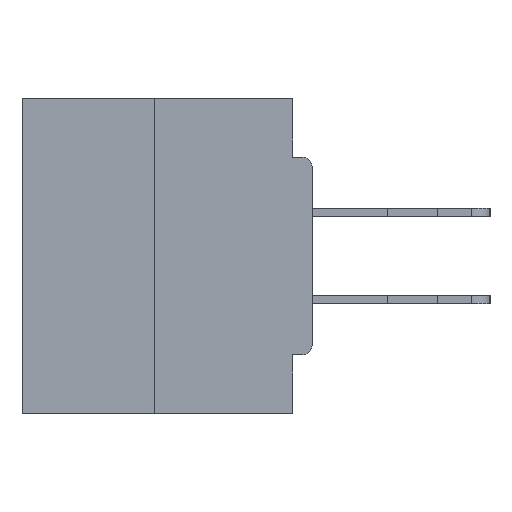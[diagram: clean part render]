
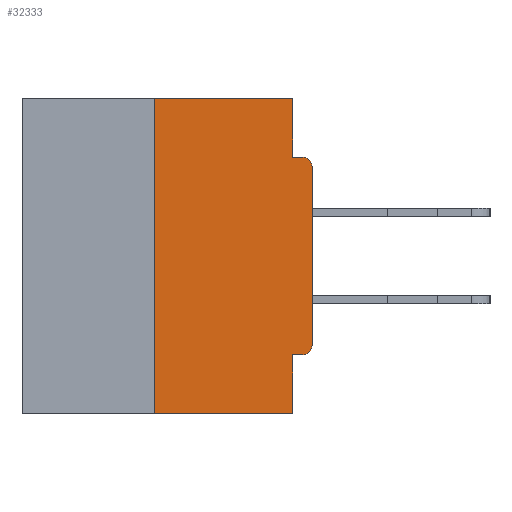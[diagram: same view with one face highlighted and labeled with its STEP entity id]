
A CAD part, left-side view. The second image highlights one B-rep face of the part: STEP entity #32333.
In plain terms, the highlighted planar face has unit normal (-1, 0, 0).
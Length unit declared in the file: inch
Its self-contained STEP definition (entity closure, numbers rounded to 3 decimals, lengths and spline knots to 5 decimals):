
#236 = CARTESIAN_POINT ( 'NONE',  ( 0., 0., -0.3915 ) ) ;
#576 = EDGE_CURVE ( 'NONE', #13654, #20772, #26147, .T. ) ;
#1003 = AXIS2_PLACEMENT_3D ( 'NONE', #36951, #21692, #18489 ) ;
#1049 = DIRECTION ( 'NONE',  ( 0., 0., 1. ) ) ;
#1581 = DIRECTION ( 'NONE',  ( 0., 0., -1. ) ) ;
#1996 = CARTESIAN_POINT ( 'NONE',  ( 0., 0.46, 0. ) ) ;
#2243 = LINE ( 'NONE', #33678, #24818 ) ;
#2298 = CARTESIAN_POINT ( 'NONE',  ( 0., 0.25, -0.5 ) ) ;
#2700 = FACE_OUTER_BOUND ( 'NONE', #12124, .T. ) ;
#2946 = VECTOR ( 'NONE', #6244, 39.37008 ) ;
#3022 = CARTESIAN_POINT ( 'NONE',  ( 0., 0.46, -0.5 ) ) ;
#3078 = LINE ( 'NONE', #3022, #37102 ) ;
#6244 = DIRECTION ( 'NONE',  ( 0., 1., 0. ) ) ;
#6319 = CARTESIAN_POINT ( 'NONE',  ( 0., 0.031, 0. ) ) ;
#6423 = DIRECTION ( 'NONE',  ( 0., 0., -1. ) ) ;
#7347 = CARTESIAN_POINT ( 'NONE',  ( 0., 0.46, 0. ) ) ;
#7908 = ORIENTED_EDGE ( 'NONE', *, *, #17415, .F. ) ;
#8770 = VERTEX_POINT ( 'NONE', #2298 ) ;
#9186 = DIRECTION ( 'NONE',  ( 0., 0., 1. ) ) ;
#9781 = CARTESIAN_POINT ( 'NONE',  ( 0., 0.031, -0.4065 ) ) ;
#10507 = VECTOR ( 'NONE', #1049, 39.37008 ) ;
#10879 = CARTESIAN_POINT ( 'NONE',  ( 0., 0., -0.1085 ) ) ;
#11119 = VECTOR ( 'NONE', #9186, 39.37008 ) ;
#11403 = ORIENTED_EDGE ( 'NONE', *, *, #34003, .F. ) ;
#11912 = CARTESIAN_POINT ( 'NONE',  ( 0., 0., 0. ) ) ;
#12124 = EDGE_LOOP ( 'NONE', ( #12538, #17332, #17091, #23481, #7908, #25326, #17087, #36339, #18971, #11403 ) ) ;
#12354 = CARTESIAN_POINT ( 'NONE',  ( 0., 0.015, -0.4065 ) ) ;
#12538 = ORIENTED_EDGE ( 'NONE', *, *, #32303, .F. ) ;
#13034 = CARTESIAN_POINT ( 'NONE',  ( 0., 0.031, -0.5 ) ) ;
#13177 = CARTESIAN_POINT ( 'NONE',  ( 0., 0.25, 0. ) ) ;
#13601 = VECTOR ( 'NONE', #29864, 39.37008 ) ;
#13654 = VERTEX_POINT ( 'NONE', #12354 ) ;
#15866 = DIRECTION ( 'NONE',  ( -1., 0., 0. ) ) ;
#16468 = EDGE_CURVE ( 'NONE', #20772, #22995, #36962, .T. ) ;
#17087 = ORIENTED_EDGE ( 'NONE', *, *, #16468, .T. ) ;
#17091 = ORIENTED_EDGE ( 'NONE', *, *, #37203, .T. ) ;
#17332 = ORIENTED_EDGE ( 'NONE', *, *, #24088, .F. ) ;
#17415 = EDGE_CURVE ( 'NONE', #13654, #19647, #22610, .T. ) ;
#17559 = CARTESIAN_POINT ( 'NONE',  ( 0., 0.031, -0.0935 ) ) ;
#18095 = VERTEX_POINT ( 'NONE', #22117 ) ;
#18348 = VERTEX_POINT ( 'NONE', #17559 ) ;
#18489 = DIRECTION ( 'NONE',  ( 0., 0., -1. ) ) ;
#18971 = ORIENTED_EDGE ( 'NONE', *, *, #31048, .F. ) ;
#19647 = VERTEX_POINT ( 'NONE', #9781 ) ;
#20772 = VERTEX_POINT ( 'NONE', #236 ) ;
#21510 = EDGE_CURVE ( 'NONE', #22995, #26286, #38523, .T. ) ;
#21692 = DIRECTION ( 'NONE',  ( -1., 0., 0. ) ) ;
#22117 = CARTESIAN_POINT ( 'NONE',  ( 0., 0.25, 0. ) ) ;
#22342 = VECTOR ( 'NONE', #37762, 39.37008 ) ;
#22610 = LINE ( 'NONE', #25053, #2946 ) ;
#22716 = VERTEX_POINT ( 'NONE', #37115 ) ;
#22810 = LINE ( 'NONE', #13034, #23332 ) ;
#22995 = VERTEX_POINT ( 'NONE', #10879 ) ;
#23332 = VECTOR ( 'NONE', #6423, 39.37008 ) ;
#23459 = AXIS2_PLACEMENT_3D ( 'NONE', #24862, #15866, #37273 ) ;
#23481 = ORIENTED_EDGE ( 'NONE', *, *, #32113, .F. ) ;
#23696 = LINE ( 'NONE', #29054, #13601 ) ;
#24088 = EDGE_CURVE ( 'NONE', #8770, #18095, #26830, .T. ) ;
#24818 = VECTOR ( 'NONE', #28049, 39.37008 ) ;
#24862 = CARTESIAN_POINT ( 'NONE',  ( 0., 0.015, -0.1085 ) ) ;
#25053 = CARTESIAN_POINT ( 'NONE',  ( 0., 0., -0.4065 ) ) ;
#25326 = ORIENTED_EDGE ( 'NONE', *, *, #576, .T. ) ;
#25369 = CARTESIAN_POINT ( 'NONE',  ( 0., 0.015, -0.0935 ) ) ;
#26106 = VERTEX_POINT ( 'NONE', #6319 ) ;
#26147 = CIRCLE ( 'NONE', #1003, 0.015 ) ;
#26286 = VERTEX_POINT ( 'NONE', #25369 ) ;
#26830 = LINE ( 'NONE', #13177, #10507 ) ;
#28049 = DIRECTION ( 'NONE',  ( 0., -1., 0. ) ) ;
#28086 = LINE ( 'NONE', #7347, #22342 ) ;
#29054 = CARTESIAN_POINT ( 'NONE',  ( 0., 0.031, 0. ) ) ;
#29227 = DIRECTION ( 'NONE',  ( 1., 0., 0. ) ) ;
#29864 = DIRECTION ( 'NONE',  ( 0., 0., -1. ) ) ;
#31048 = EDGE_CURVE ( 'NONE', #18348, #26286, #2243, .T. ) ;
#32030 = AXIS2_PLACEMENT_3D ( 'NONE', #1996, #29227, #1581 ) ;
#32113 = EDGE_CURVE ( 'NONE', #19647, #22716, #22810, .T. ) ;
#32152 = PLANE ( 'NONE',  #32030 ) ;
#32303 = EDGE_CURVE ( 'NONE', #18095, #26106, #28086, .T. ) ;
#32333 = ADVANCED_FACE ( 'NONE', ( #2700 ), #32152, .F. ) ;
#33678 = CARTESIAN_POINT ( 'NONE',  ( 0., 0., -0.0935 ) ) ;
#34003 = EDGE_CURVE ( 'NONE', #26106, #18348, #23696, .T. ) ;
#36339 = ORIENTED_EDGE ( 'NONE', *, *, #21510, .T. ) ;
#36396 = DIRECTION ( 'NONE',  ( 0., -1., 0. ) ) ;
#36951 = CARTESIAN_POINT ( 'NONE',  ( 0., 0.015, -0.3915 ) ) ;
#36962 = LINE ( 'NONE', #11912, #11119 ) ;
#37102 = VECTOR ( 'NONE', #36396, 39.37008 ) ;
#37115 = CARTESIAN_POINT ( 'NONE',  ( 0., 0.031, -0.5 ) ) ;
#37203 = EDGE_CURVE ( 'NONE', #8770, #22716, #3078, .T. ) ;
#37273 = DIRECTION ( 'NONE',  ( 0., 0., -1. ) ) ;
#37762 = DIRECTION ( 'NONE',  ( 0., -1., 0. ) ) ;
#38523 = CIRCLE ( 'NONE', #23459, 0.015 ) ;
